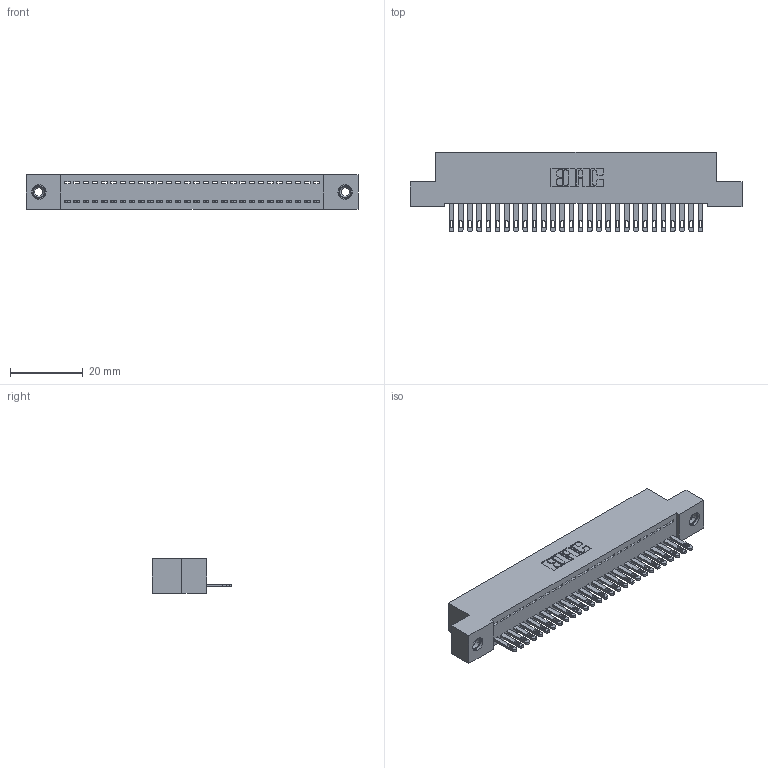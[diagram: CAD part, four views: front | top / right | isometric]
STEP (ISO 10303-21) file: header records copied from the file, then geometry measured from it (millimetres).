
FILE_DESCRIPTION (( 'STEP AP203' ), '1' );
FILE_NAME ('892-028-500-108.STEP', '2020-09-21T14:52:21', ( '' ), ( '' ), 'SwSTEP 2.0', 'SolidWorks 2020', '' );
FILE_SCHEMA (( 'CONFIG_CONTROL_DESIGN' ));
Length unit declared in the file: inch
Products named in the file (4): 842 Part_TI; 892-028-500-108; 345-292-001_345-293-100; 345-250-001_345-250-003-102
Assembly tree (31 placements, depth 2):
  892-028-500-108
    842 Part_TI
    345-292-001_345-293-100  x28
    345-250-001_345-250-003-102  x2
Bounding box: 91.44 x 21.85 x 9.4 mm (x, y, z)
Volume: 7977.5 mm3; surface area: 11526.2 mm2
Topology: 31 solids, 31 shells, 1682 faces, 5139 edges, 3418 vertices
Faces by surface type: plane 1106, cylinder 560, cone 12, torus 4
Entity records: 19912 total; most frequent: CARTESIAN_POINT 3417, ORIENTED_EDGE 3374, DIRECTION 2945, EDGE_CURVE 1687, VECTOR 1535, LINE 1535, VERTEX_POINT 1120, AXIS2_PLACEMENT_3D 705
